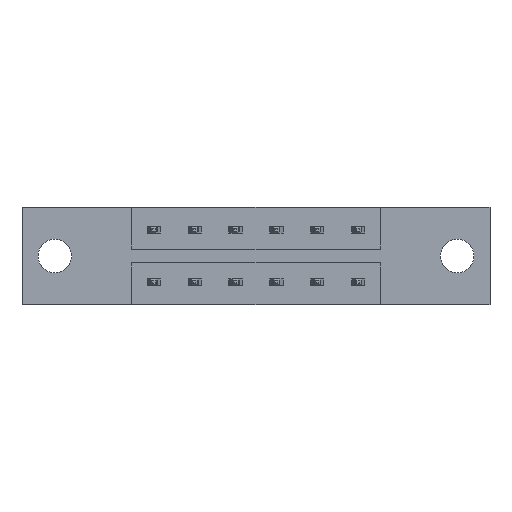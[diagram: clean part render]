
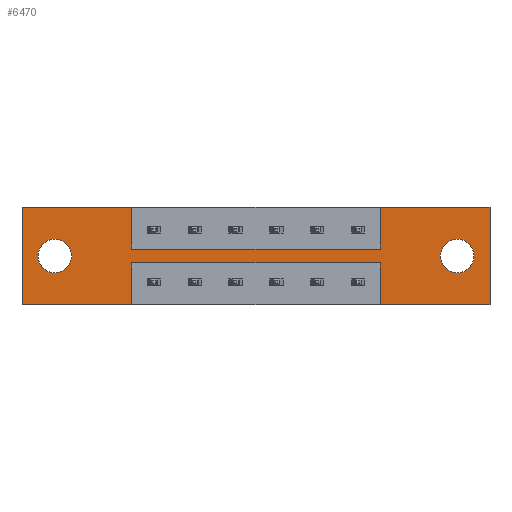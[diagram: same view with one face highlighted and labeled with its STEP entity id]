
A CAD part, front view. The second image highlights one B-rep face of the part: STEP entity #6470.
In plain terms, the highlighted planar face has unit normal (0, -1, 0).
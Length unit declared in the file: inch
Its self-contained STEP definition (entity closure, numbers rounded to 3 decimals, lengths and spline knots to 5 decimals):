
#80 = LINE ( 'NONE', #7923, #2043 ) ;
#101 = VERTEX_POINT ( 'NONE', #4799 ) ;
#207 = DIRECTION ( 'NONE',  ( 0., 0., -1. ) ) ;
#218 = VERTEX_POINT ( 'NONE', #6914 ) ;
#273 = CARTESIAN_POINT ( 'NONE',  ( 1.784, 0., -0.37 ) ) ;
#400 = VECTOR ( 'NONE', #1687, 39.37008 ) ;
#429 = CARTESIAN_POINT ( 'NONE',  ( 0., 0., -0.37 ) ) ;
#505 = CARTESIAN_POINT ( 'NONE',  ( 0.4175, 0., -0.1585 ) ) ;
#613 = AXIS2_PLACEMENT_3D ( 'NONE', #2084, #3661, #6260 ) ;
#942 = VECTOR ( 'NONE', #3337, 39.37008 ) ;
#944 = EDGE_LOOP ( 'NONE', ( #4588, #7340 ) ) ;
#1162 = DIRECTION ( 'NONE',  ( 0., 0., -1. ) ) ;
#1170 = EDGE_CURVE ( 'NONE', #2456, #1827, #80, .T. ) ;
#1197 = VECTOR ( 'NONE', #7725, 39.37008 ) ;
#1198 = DIRECTION ( 'NONE',  ( 0., 1., 0. ) ) ;
#1220 = CARTESIAN_POINT ( 'NONE',  ( 0., 0., 0. ) ) ;
#1254 = CARTESIAN_POINT ( 'NONE',  ( 1.659, 0., -0.185 ) ) ;
#1478 = EDGE_CURVE ( 'NONE', #3437, #6029, #1688, .T. ) ;
#1635 = AXIS2_PLACEMENT_3D ( 'NONE', #1254, #1198, #1162 ) ;
#1646 = DIRECTION ( 'NONE',  ( 0., 1., 0. ) ) ;
#1651 = LINE ( 'NONE', #8389, #6885 ) ;
#1659 = EDGE_CURVE ( 'NONE', #3662, #4069, #6013, .T. ) ;
#1673 = DIRECTION ( 'NONE',  ( 0., 0., 1. ) ) ;
#1675 = DIRECTION ( 'NONE',  ( 0., 1., 0. ) ) ;
#1687 = DIRECTION ( 'NONE',  ( 1., 0., 0. ) ) ;
#1688 = LINE ( 'NONE', #8185, #8376 ) ;
#1703 = CARTESIAN_POINT ( 'NONE',  ( 0.125, 0., -0.185 ) ) ;
#1803 = EDGE_CURVE ( 'NONE', #3946, #3662, #3528, .T. ) ;
#1823 = CARTESIAN_POINT ( 'NONE',  ( 0., 0., -0.37 ) ) ;
#1827 = VERTEX_POINT ( 'NONE', #273 ) ;
#1965 = CARTESIAN_POINT ( 'NONE',  ( 0.125, 0., -0.121 ) ) ;
#2002 = EDGE_CURVE ( 'NONE', #6029, #2456, #5889, .T. ) ;
#2043 = VECTOR ( 'NONE', #7369, 39.37008 ) ;
#2084 = CARTESIAN_POINT ( 'NONE',  ( 0., 0., -0.37 ) ) ;
#2105 = PLANE ( 'NONE',  #613 ) ;
#2152 = EDGE_CURVE ( 'NONE', #101, #3928, #4769, .T. ) ;
#2236 = VECTOR ( 'NONE', #5366, 39.37008 ) ;
#2243 = VERTEX_POINT ( 'NONE', #6579 ) ;
#2428 = EDGE_CURVE ( 'NONE', #2830, #101, #4436, .T. ) ;
#2456 = VERTEX_POINT ( 'NONE', #3106 ) ;
#2469 = VERTEX_POINT ( 'NONE', #2895 ) ;
#2493 = CARTESIAN_POINT ( 'NONE',  ( 1.659, 0., -0.121 ) ) ;
#2515 = CARTESIAN_POINT ( 'NONE',  ( 0.125, 0., -0.249 ) ) ;
#2602 = FACE_BOUND ( 'NONE', #944, .T. ) ;
#2749 = VECTOR ( 'NONE', #3525, 39.37008 ) ;
#2804 = FACE_BOUND ( 'NONE', #4987, .T. ) ;
#2828 = LINE ( 'NONE', #3273, #942 ) ;
#2830 = VERTEX_POINT ( 'NONE', #7188 ) ;
#2895 = CARTESIAN_POINT ( 'NONE',  ( 1.659, 0., -0.249 ) ) ;
#3025 = EDGE_CURVE ( 'NONE', #3928, #3946, #4860, .T. ) ;
#3056 = CARTESIAN_POINT ( 'NONE',  ( 1.3665, 0., -0.1585 ) ) ;
#3058 = AXIS2_PLACEMENT_3D ( 'NONE', #5636, #1646, #6444 ) ;
#3106 = CARTESIAN_POINT ( 'NONE',  ( 1.784, 0., 0. ) ) ;
#3148 = EDGE_CURVE ( 'NONE', #4069, #2243, #5156, .T. ) ;
#3169 = DIRECTION ( 'NONE',  ( 0., 0., 1. ) ) ;
#3214 = CIRCLE ( 'NONE', #3829, 0.064 ) ;
#3273 = CARTESIAN_POINT ( 'NONE',  ( 0., 0., -0.37 ) ) ;
#3337 = DIRECTION ( 'NONE',  ( -1., 0., 0. ) ) ;
#3417 = VECTOR ( 'NONE', #4856, 39.37008 ) ;
#3437 = VERTEX_POINT ( 'NONE', #3056 ) ;
#3525 = DIRECTION ( 'NONE',  ( 0., 0., 1. ) ) ;
#3528 = LINE ( 'NONE', #429, #8451 ) ;
#3554 = CIRCLE ( 'NONE', #3058, 0.064 ) ;
#3579 = DIRECTION ( 'NONE',  ( 0., 0., -1. ) ) ;
#3626 = DIRECTION ( 'NONE',  ( 0., 1., 0. ) ) ;
#3661 = DIRECTION ( 'NONE',  ( 0., -1., 0. ) ) ;
#3662 = VERTEX_POINT ( 'NONE', #1823 ) ;
#3675 = VERTEX_POINT ( 'NONE', #1965 ) ;
#3684 = EDGE_CURVE ( 'NONE', #3675, #6110, #8016, .T. ) ;
#3770 = CARTESIAN_POINT ( 'NONE',  ( 1.659, 0., -0.185 ) ) ;
#3829 = AXIS2_PLACEMENT_3D ( 'NONE', #3770, #3626, #3579 ) ;
#3928 = VERTEX_POINT ( 'NONE', #6127 ) ;
#3946 = VERTEX_POINT ( 'NONE', #4960 ) ;
#4069 = VERTEX_POINT ( 'NONE', #1220 ) ;
#4202 = CARTESIAN_POINT ( 'NONE',  ( 1.3665, 0., -0.2115 ) ) ;
#4293 = EDGE_CURVE ( 'NONE', #2243, #218, #4548, .T. ) ;
#4436 = LINE ( 'NONE', #4202, #2749 ) ;
#4548 = LINE ( 'NONE', #505, #7865 ) ;
#4588 = ORIENTED_EDGE ( 'NONE', *, *, #3684, .T. ) ;
#4626 = ORIENTED_EDGE ( 'NONE', *, *, #1659, .F. ) ;
#4688 = ORIENTED_EDGE ( 'NONE', *, *, #3025, .F. ) ;
#4716 = DIRECTION ( 'NONE',  ( -1., 0., 0. ) ) ;
#4769 = LINE ( 'NONE', #7745, #1197 ) ;
#4799 = CARTESIAN_POINT ( 'NONE',  ( 1.3665, 0., -0.2115 ) ) ;
#4832 = ORIENTED_EDGE ( 'NONE', *, *, #5190, .F. ) ;
#4856 = DIRECTION ( 'NONE',  ( 1., 0., 0. ) ) ;
#4860 = LINE ( 'NONE', #5916, #7944 ) ;
#4941 = VERTEX_POINT ( 'NONE', #2493 ) ;
#4960 = CARTESIAN_POINT ( 'NONE',  ( 0.4175, 0., -0.37 ) ) ;
#4987 = EDGE_LOOP ( 'NONE', ( #6818, #6875 ) ) ;
#5016 = CARTESIAN_POINT ( 'NONE',  ( 0., 0., 0. ) ) ;
#5020 = EDGE_CURVE ( 'NONE', #4941, #2469, #6986, .T. ) ;
#5128 = ORIENTED_EDGE ( 'NONE', *, *, #2002, .F. ) ;
#5156 = LINE ( 'NONE', #5016, #3417 ) ;
#5190 = EDGE_CURVE ( 'NONE', #218, #3437, #1651, .T. ) ;
#5240 = ORIENTED_EDGE ( 'NONE', *, *, #2152, .F. ) ;
#5305 = EDGE_CURVE ( 'NONE', #1827, #2830, #2828, .T. ) ;
#5314 = EDGE_CURVE ( 'NONE', #2469, #4941, #3214, .T. ) ;
#5321 = CARTESIAN_POINT ( 'NONE',  ( 0., 0., 0. ) ) ;
#5366 = DIRECTION ( 'NONE',  ( 0., 0., 1. ) ) ;
#5506 = AXIS2_PLACEMENT_3D ( 'NONE', #1703, #1675, #1673 ) ;
#5636 = CARTESIAN_POINT ( 'NONE',  ( 0.125, 0., -0.185 ) ) ;
#5695 = CARTESIAN_POINT ( 'NONE',  ( 1.3665, 0., 0. ) ) ;
#5711 = DIRECTION ( 'NONE',  ( 0., 0., -1. ) ) ;
#5889 = LINE ( 'NONE', #7505, #400 ) ;
#5916 = CARTESIAN_POINT ( 'NONE',  ( 0.4175, 0., -0.2115 ) ) ;
#6013 = LINE ( 'NONE', #5321, #2236 ) ;
#6029 = VERTEX_POINT ( 'NONE', #5695 ) ;
#6110 = VERTEX_POINT ( 'NONE', #2515 ) ;
#6127 = CARTESIAN_POINT ( 'NONE',  ( 0.4175, 0., -0.2115 ) ) ;
#6260 = DIRECTION ( 'NONE',  ( 0., 0., -1. ) ) ;
#6319 = ORIENTED_EDGE ( 'NONE', *, *, #4293, .F. ) ;
#6325 = ORIENTED_EDGE ( 'NONE', *, *, #3148, .F. ) ;
#6334 = ORIENTED_EDGE ( 'NONE', *, *, #1803, .F. ) ;
#6444 = DIRECTION ( 'NONE',  ( 0., 0., 1. ) ) ;
#6470 = ADVANCED_FACE ( 'NONE', ( #2804, #2602, #7836 ), #2105, .T. ) ;
#6579 = CARTESIAN_POINT ( 'NONE',  ( 0.4175, 0., 0. ) ) ;
#6818 = ORIENTED_EDGE ( 'NONE', *, *, #5020, .T. ) ;
#6875 = ORIENTED_EDGE ( 'NONE', *, *, #5314, .T. ) ;
#6885 = VECTOR ( 'NONE', #7993, 39.37008 ) ;
#6914 = CARTESIAN_POINT ( 'NONE',  ( 0.4175, 0., -0.1585 ) ) ;
#6923 = ORIENTED_EDGE ( 'NONE', *, *, #5305, .F. ) ;
#6986 = CIRCLE ( 'NONE', #1635, 0.064 ) ;
#7027 = ORIENTED_EDGE ( 'NONE', *, *, #2428, .F. ) ;
#7188 = CARTESIAN_POINT ( 'NONE',  ( 1.3665, 0., -0.37 ) ) ;
#7200 = ORIENTED_EDGE ( 'NONE', *, *, #1170, .F. ) ;
#7340 = ORIENTED_EDGE ( 'NONE', *, *, #8193, .T. ) ;
#7369 = DIRECTION ( 'NONE',  ( 0., 0., -1. ) ) ;
#7505 = CARTESIAN_POINT ( 'NONE',  ( 0., 0., 0. ) ) ;
#7602 = ORIENTED_EDGE ( 'NONE', *, *, #1478, .F. ) ;
#7725 = DIRECTION ( 'NONE',  ( -1., 0., 0. ) ) ;
#7745 = CARTESIAN_POINT ( 'NONE',  ( 0.4175, 0., -0.2115 ) ) ;
#7836 = FACE_OUTER_BOUND ( 'NONE', #8103, .T. ) ;
#7865 = VECTOR ( 'NONE', #207, 39.37008 ) ;
#7923 = CARTESIAN_POINT ( 'NONE',  ( 1.784, 0., 0. ) ) ;
#7944 = VECTOR ( 'NONE', #5711, 39.37008 ) ;
#7993 = DIRECTION ( 'NONE',  ( 1., 0., 0. ) ) ;
#8016 = CIRCLE ( 'NONE', #5506, 0.064 ) ;
#8103 = EDGE_LOOP ( 'NONE', ( #7027, #6923, #7200, #5128, #7602, #4832, #6319, #6325, #4626, #6334, #4688, #5240 ) ) ;
#8185 = CARTESIAN_POINT ( 'NONE',  ( 1.3665, 0., -0.1585 ) ) ;
#8193 = EDGE_CURVE ( 'NONE', #6110, #3675, #3554, .T. ) ;
#8376 = VECTOR ( 'NONE', #3169, 39.37008 ) ;
#8389 = CARTESIAN_POINT ( 'NONE',  ( 0.4175, 0., -0.1585 ) ) ;
#8451 = VECTOR ( 'NONE', #4716, 39.37008 ) ;
